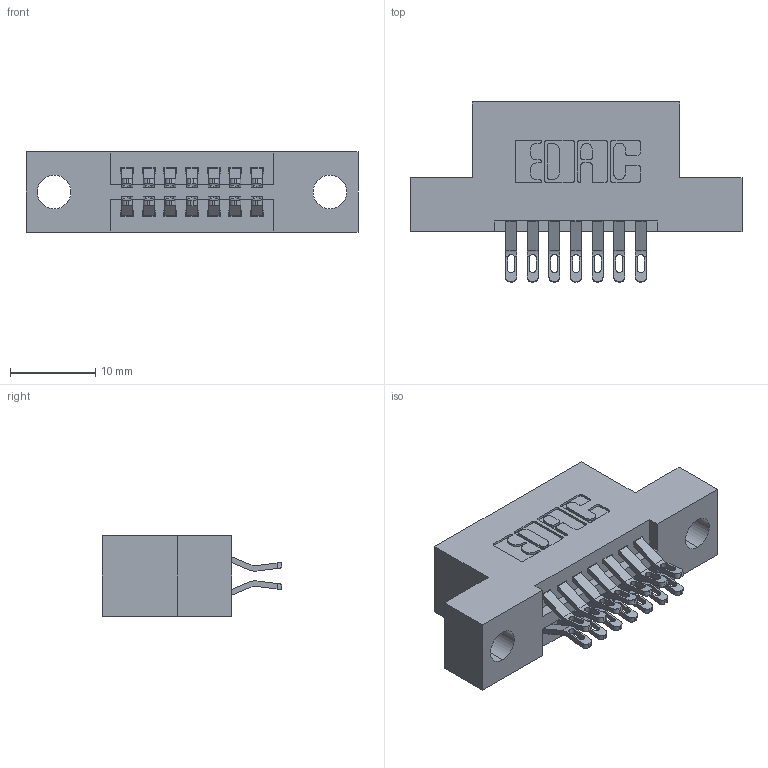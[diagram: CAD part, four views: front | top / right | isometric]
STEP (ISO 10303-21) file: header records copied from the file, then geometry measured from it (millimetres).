
FILE_DESCRIPTION (( 'STEP AP203' ), '1' );
FILE_NAME ('395-014-555-204.STEP', '2021-06-14T18:01:34', ( '' ), ( '' ), 'SwSTEP 2.0', 'SolidWorks 2020', '' );
FILE_SCHEMA (( 'CONFIG_CONTROL_DESIGN' ));
Length unit declared in the file: inch
Products named in the file (3): 345-292-001_555 Tail; 395-014-555-204; 345 Part_Flush Mounting Lugs - 0.156 Dia-TI
Assembly tree (15 placements, depth 2):
  395-014-555-204
    345 Part_Flush Mounting Lugs - 0.156 Dia-TI
    345-292-001_555 Tail  x14
Bounding box: 38.99 x 21.13 x 9.4 mm (x, y, z)
Volume: 3397.2 mm3; surface area: 4336.6 mm2
Topology: 15 solids, 15 shells, 924 faces, 2855 edges, 1902 vertices
Faces by surface type: plane 528, cylinder 396
Entity records: 10949 total; most frequent: CARTESIAN_POINT 1908, ORIENTED_EDGE 1810, DIRECTION 1693, EDGE_CURVE 905, VECTOR 725, LINE 725, VERTEX_POINT 602, AXIS2_PLACEMENT_3D 484
